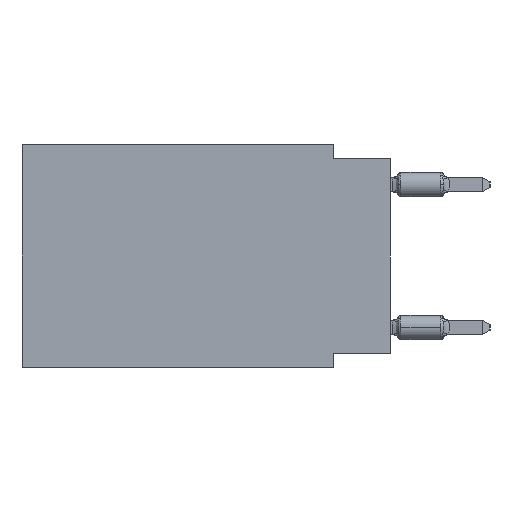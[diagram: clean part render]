
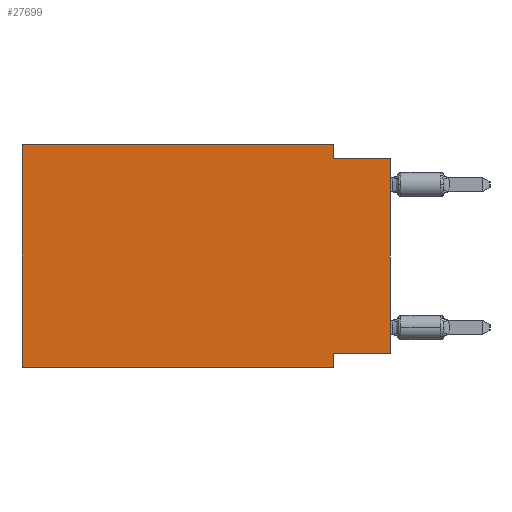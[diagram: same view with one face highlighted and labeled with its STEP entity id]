
A CAD part, left-side view. The second image highlights one B-rep face of the part: STEP entity #27699.
In plain terms, the highlighted planar face has unit normal (-1, 0, 0).
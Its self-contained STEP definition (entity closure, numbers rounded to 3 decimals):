
#2279 = LINE ( 'NONE', #48031, #31748 ) ;
#2463 = EDGE_LOOP ( 'NONE', ( #25633, #26855, #30755, #26467, #8947, #32454, #2640, #20784 ) ) ;
#2640 = ORIENTED_EDGE ( 'NONE', *, *, #24588, .F. ) ;
#4532 = CARTESIAN_POINT ( 'NONE',  ( 0., 0., -9.271 ) ) ;
#4968 = VERTEX_POINT ( 'NONE', #19655 ) ;
#5137 = CARTESIAN_POINT ( 'NONE',  ( 0., 2.54, -9.906 ) ) ;
#6394 = CARTESIAN_POINT ( 'NONE',  ( 0., 2.54, 0. ) ) ;
#7936 = EDGE_CURVE ( 'NONE', #14452, #40140, #40653, .T. ) ;
#8285 = LINE ( 'NONE', #4532, #20458 ) ;
#8947 = ORIENTED_EDGE ( 'NONE', *, *, #45065, .F. ) ;
#9659 = DIRECTION ( 'NONE',  ( 0., -1., 0. ) ) ;
#9777 = LINE ( 'NONE', #48778, #20558 ) ;
#10016 = DIRECTION ( 'NONE',  ( 0., 0., 1. ) ) ;
#10890 = FACE_OUTER_BOUND ( 'NONE', #2463, .T. ) ;
#12004 = LINE ( 'NONE', #43910, #34962 ) ;
#13271 = DIRECTION ( 'NONE',  ( 0., -1., 0. ) ) ;
#14452 = VERTEX_POINT ( 'NONE', #20748 ) ;
#15811 = LINE ( 'NONE', #31084, #23096 ) ;
#17588 = VECTOR ( 'NONE', #13271, 1000. ) ;
#17734 = EDGE_CURVE ( 'NONE', #4968, #48546, #20284, .T. ) ;
#19655 = CARTESIAN_POINT ( 'NONE',  ( 0., 16.383, -9.906 ) ) ;
#20284 = LINE ( 'NONE', #43311, #17588 ) ;
#20458 = VECTOR ( 'NONE', #46774, 1000. ) ;
#20558 = VECTOR ( 'NONE', #48263, 1000. ) ;
#20748 = CARTESIAN_POINT ( 'NONE',  ( 0., 2.54, 0. ) ) ;
#20784 = ORIENTED_EDGE ( 'NONE', *, *, #41772, .F. ) ;
#21632 = DIRECTION ( 'NONE',  ( 0., 0., -1. ) ) ;
#22063 = VECTOR ( 'NONE', #46110, 1000. ) ;
#22125 = DIRECTION ( 'NONE',  ( 0., 0., -1. ) ) ;
#23096 = VECTOR ( 'NONE', #49326, 1000. ) ;
#24309 = CARTESIAN_POINT ( 'NONE',  ( 0., 2.54, -0.635 ) ) ;
#24588 = EDGE_CURVE ( 'NONE', #46826, #48546, #31117, .T. ) ;
#25633 = ORIENTED_EDGE ( 'NONE', *, *, #45186, .T. ) ;
#26467 = ORIENTED_EDGE ( 'NONE', *, *, #27579, .F. ) ;
#26855 = ORIENTED_EDGE ( 'NONE', *, *, #29584, .F. ) ;
#27579 = EDGE_CURVE ( 'NONE', #39886, #14452, #12004, .T. ) ;
#27587 = CARTESIAN_POINT ( 'NONE',  ( 0., 0., -0.635 ) ) ;
#27699 = ADVANCED_FACE ( 'NONE', ( #10890 ), #33133, .F. ) ;
#29584 = EDGE_CURVE ( 'NONE', #40140, #41345, #15811, .T. ) ;
#29885 = CARTESIAN_POINT ( 'NONE',  ( 0., 16.383, 0. ) ) ;
#30755 = ORIENTED_EDGE ( 'NONE', *, *, #7936, .F. ) ;
#31084 = CARTESIAN_POINT ( 'NONE',  ( 0., 0., -0.635 ) ) ;
#31117 = LINE ( 'NONE', #42116, #22063 ) ;
#31748 = VECTOR ( 'NONE', #10016, 1000. ) ;
#32454 = ORIENTED_EDGE ( 'NONE', *, *, #17734, .T. ) ;
#32968 = CARTESIAN_POINT ( 'NONE',  ( 0., 2.54, -9.271 ) ) ;
#33133 = PLANE ( 'NONE',  #38976 ) ;
#34962 = VECTOR ( 'NONE', #9659, 1000. ) ;
#38443 = VECTOR ( 'NONE', #21632, 1000. ) ;
#38976 = AXIS2_PLACEMENT_3D ( 'NONE', #29885, #48893, #22125 ) ;
#39886 = VERTEX_POINT ( 'NONE', #41116 ) ;
#40140 = VERTEX_POINT ( 'NONE', #24309 ) ;
#40653 = LINE ( 'NONE', #6394, #38443 ) ;
#40829 = CARTESIAN_POINT ( 'NONE',  ( 0., 0., -9.271 ) ) ;
#41116 = CARTESIAN_POINT ( 'NONE',  ( 0., 16.383, 0. ) ) ;
#41345 = VERTEX_POINT ( 'NONE', #27587 ) ;
#41772 = EDGE_CURVE ( 'NONE', #48027, #46826, #8285, .T. ) ;
#42116 = CARTESIAN_POINT ( 'NONE',  ( 0., 2.54, -9.906 ) ) ;
#43311 = CARTESIAN_POINT ( 'NONE',  ( 0., 16.383, -9.906 ) ) ;
#43910 = CARTESIAN_POINT ( 'NONE',  ( 0., 16.383, 0. ) ) ;
#45065 = EDGE_CURVE ( 'NONE', #4968, #39886, #9777, .T. ) ;
#45186 = EDGE_CURVE ( 'NONE', #48027, #41345, #2279, .T. ) ;
#46110 = DIRECTION ( 'NONE',  ( 0., 0., -1. ) ) ;
#46774 = DIRECTION ( 'NONE',  ( 0., 1., 0. ) ) ;
#46826 = VERTEX_POINT ( 'NONE', #32968 ) ;
#48027 = VERTEX_POINT ( 'NONE', #40829 ) ;
#48031 = CARTESIAN_POINT ( 'NONE',  ( 0., 0., 0. ) ) ;
#48263 = DIRECTION ( 'NONE',  ( 0., 0., 1. ) ) ;
#48546 = VERTEX_POINT ( 'NONE', #5137 ) ;
#48778 = CARTESIAN_POINT ( 'NONE',  ( 0., 16.383, 0. ) ) ;
#48893 = DIRECTION ( 'NONE',  ( 1., 0., 0. ) ) ;
#49326 = DIRECTION ( 'NONE',  ( 0., -1., 0. ) ) ;
